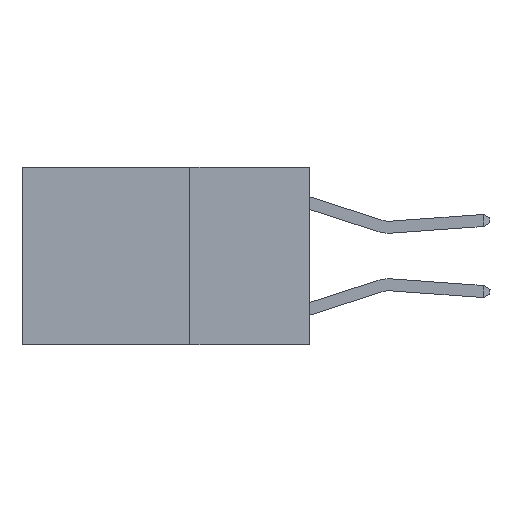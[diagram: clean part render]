
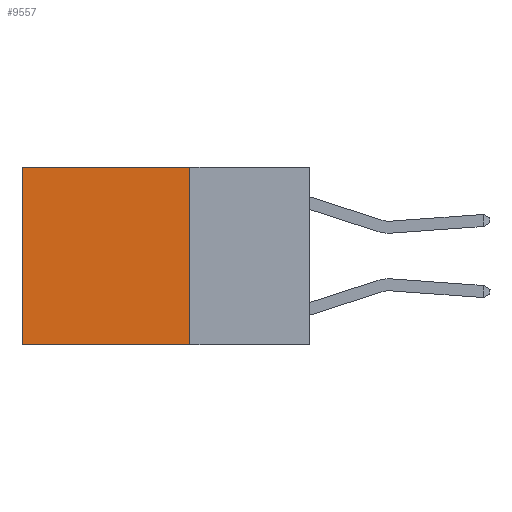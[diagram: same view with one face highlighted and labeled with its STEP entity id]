
A CAD part, left-side view. The second image highlights one B-rep face of the part: STEP entity #9557.
In plain terms, the highlighted planar face has unit normal (-1, 0, 0).
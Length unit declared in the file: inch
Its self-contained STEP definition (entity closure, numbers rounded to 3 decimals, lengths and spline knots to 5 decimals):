
#193 = LINE ( 'NONE', #686, #5539 ) ;
#297 = VERTEX_POINT ( 'NONE', #13143 ) ;
#686 = CARTESIAN_POINT ( 'NONE',  ( 0.2625, 0.25, 0. ) ) ;
#798 = DIRECTION ( 'NONE',  ( 0., 1., 0. ) ) ;
#1437 = PLANE ( 'NONE',  #24185 ) ;
#1820 = ORIENTED_EDGE ( 'NONE', *, *, #2117, .T. ) ;
#2117 = EDGE_CURVE ( 'NONE', #6505, #23334, #3768, .T. ) ;
#2739 = ORIENTED_EDGE ( 'NONE', *, *, #8648, .F. ) ;
#3768 = LINE ( 'NONE', #13427, #14227 ) ;
#3973 = EDGE_CURVE ( 'NONE', #19577, #297, #18933, .T. ) ;
#4188 = ORIENTED_EDGE ( 'NONE', *, *, #3973, .F. ) ;
#5277 = CARTESIAN_POINT ( 'NONE',  ( 0.2625, 0.6, 0. ) ) ;
#5539 = VECTOR ( 'NONE', #10554, 39.37008 ) ;
#6505 = VERTEX_POINT ( 'NONE', #22032 ) ;
#7441 = DIRECTION ( 'NONE',  ( 0., 0., -1. ) ) ;
#8648 = EDGE_CURVE ( 'NONE', #6505, #19577, #193, .T. ) ;
#9149 = VECTOR ( 'NONE', #17048, 39.37008 ) ;
#9557 = ADVANCED_FACE ( 'NONE', ( #12368 ), #1437, .F. ) ;
#10554 = DIRECTION ( 'NONE',  ( 0., 0., -1. ) ) ;
#10626 = ORIENTED_EDGE ( 'NONE', *, *, #13554, .T. ) ;
#10659 = CARTESIAN_POINT ( 'NONE',  ( 0.2625, 0.25, -0.37 ) ) ;
#12368 = FACE_OUTER_BOUND ( 'NONE', #23600, .T. ) ;
#13143 = CARTESIAN_POINT ( 'NONE',  ( 0.2625, 0.6, -0.37 ) ) ;
#13287 = CARTESIAN_POINT ( 'NONE',  ( 0.2625, 0.25, 0. ) ) ;
#13427 = CARTESIAN_POINT ( 'NONE',  ( 0.2625, 0.25, 0. ) ) ;
#13554 = EDGE_CURVE ( 'NONE', #23334, #297, #24730, .T. ) ;
#13720 = VECTOR ( 'NONE', #798, 39.37008 ) ;
#14227 = VECTOR ( 'NONE', #15394, 39.37008 ) ;
#15394 = DIRECTION ( 'NONE',  ( 0., 1., 0. ) ) ;
#16487 = CARTESIAN_POINT ( 'NONE',  ( 0.2625, 0.6, 0. ) ) ;
#17048 = DIRECTION ( 'NONE',  ( 0., 0., -1. ) ) ;
#18933 = LINE ( 'NONE', #10659, #13720 ) ;
#19189 = DIRECTION ( 'NONE',  ( 1., 0., 0. ) ) ;
#19577 = VERTEX_POINT ( 'NONE', #22310 ) ;
#22032 = CARTESIAN_POINT ( 'NONE',  ( 0.2625, 0.25, 0. ) ) ;
#22310 = CARTESIAN_POINT ( 'NONE',  ( 0.2625, 0.25, -0.37 ) ) ;
#23334 = VERTEX_POINT ( 'NONE', #16487 ) ;
#23600 = EDGE_LOOP ( 'NONE', ( #10626, #4188, #2739, #1820 ) ) ;
#24185 = AXIS2_PLACEMENT_3D ( 'NONE', #13287, #19189, #7441 ) ;
#24730 = LINE ( 'NONE', #5277, #9149 ) ;
